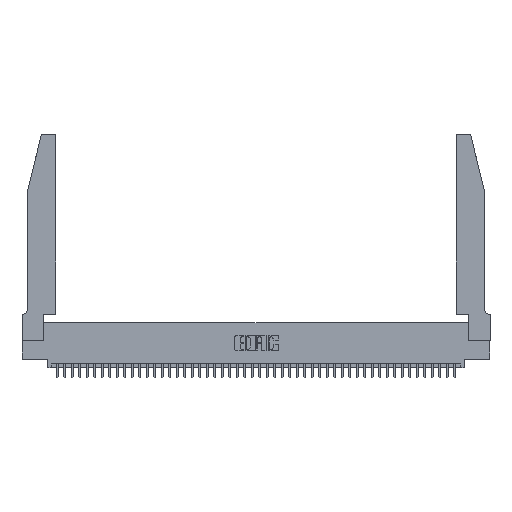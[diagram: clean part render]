
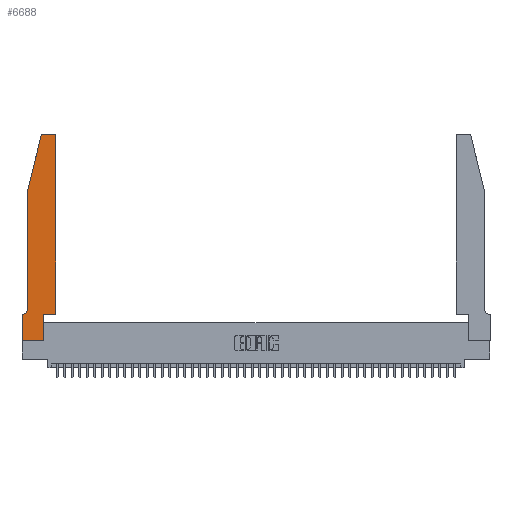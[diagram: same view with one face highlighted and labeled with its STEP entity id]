
A CAD part, top view. The second image highlights one B-rep face of the part: STEP entity #6688.
In plain terms, the highlighted planar face has unit normal (0, 0, 1).
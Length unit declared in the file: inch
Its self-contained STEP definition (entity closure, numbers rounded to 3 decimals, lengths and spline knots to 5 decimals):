
#285 = CARTESIAN_POINT ( 'NONE',  ( 0.0755, 0.35, 0.37 ) ) ;
#939 = VERTEX_POINT ( 'NONE', #20002 ) ;
#1059 = VERTEX_POINT ( 'NONE', #38170 ) ;
#1224 = DIRECTION ( 'NONE',  ( 1., 0., 0. ) ) ;
#1746 = DIRECTION ( 'NONE',  ( 0., -1., 0. ) ) ;
#1923 = VERTEX_POINT ( 'NONE', #30181 ) ;
#2543 = DIRECTION ( 'NONE',  ( 0., 0., 1. ) ) ;
#3639 = CARTESIAN_POINT ( 'NONE',  ( 0.4505, 0.35, 0.37 ) ) ;
#5218 = CARTESIAN_POINT ( 'NONE',  ( 0., 0., 0.37 ) ) ;
#5653 = CARTESIAN_POINT ( 'NONE',  ( 0., 0.35, 0.37 ) ) ;
#5811 = EDGE_CURVE ( 'NONE', #19131, #30120, #33323, .T. ) ;
#5924 = VECTOR ( 'NONE', #8191, 39.37008 ) ;
#6091 = DIRECTION ( 'NONE',  ( 1., 0., 0. ) ) ;
#6151 = EDGE_CURVE ( 'NONE', #26270, #1059, #14539, .T. ) ;
#6517 = CARTESIAN_POINT ( 'NONE',  ( 0.284, 2.75, 0.37 ) ) ;
#6688 = ADVANCED_FACE ( 'NONE', ( #35357 ), #9318, .T. ) ;
#7114 = CARTESIAN_POINT ( 'NONE',  ( 0.0055, 0.42, 0.37 ) ) ;
#7132 = EDGE_CURVE ( 'NONE', #28890, #1923, #33712, .T. ) ;
#7507 = VECTOR ( 'NONE', #43722, 39.37008 ) ;
#7751 = ORIENTED_EDGE ( 'NONE', *, *, #31912, .T. ) ;
#8060 = ORIENTED_EDGE ( 'NONE', *, *, #38276, .T. ) ;
#8191 = DIRECTION ( 'NONE',  ( -1., 0., 0. ) ) ;
#8782 = CARTESIAN_POINT ( 'NONE',  ( 0., 0.35, 0.37 ) ) ;
#8792 = CARTESIAN_POINT ( 'NONE',  ( 0.4505, 2.72, 0.37 ) ) ;
#9318 = PLANE ( 'NONE',  #44135 ) ;
#9440 = VERTEX_POINT ( 'NONE', #23619 ) ;
#10139 = ORIENTED_EDGE ( 'NONE', *, *, #34763, .T. ) ;
#10214 = EDGE_CURVE ( 'NONE', #1923, #26270, #35116, .T. ) ;
#10423 = EDGE_CURVE ( 'NONE', #27678, #28890, #35073, .T. ) ;
#11767 = EDGE_CURVE ( 'NONE', #939, #9440, #40480, .T. ) ;
#12147 = CARTESIAN_POINT ( 'NONE',  ( 0.0755, 2., 0.37 ) ) ;
#13670 = ORIENTED_EDGE ( 'NONE', *, *, #6151, .T. ) ;
#13792 = CARTESIAN_POINT ( 'NONE',  ( 0.0755, 2., 0.37 ) ) ;
#14059 = VERTEX_POINT ( 'NONE', #31666 ) ;
#14539 = CIRCLE ( 'NONE', #23484, 0.03 ) ;
#14559 = VECTOR ( 'NONE', #45145, 39.37008 ) ;
#15178 = ORIENTED_EDGE ( 'NONE', *, *, #5811, .T. ) ;
#15927 = VECTOR ( 'NONE', #21451, 39.37008 ) ;
#16009 = CARTESIAN_POINT ( 'NONE',  ( 0.4505, 0.35, 0.37 ) ) ;
#16106 = ORIENTED_EDGE ( 'NONE', *, *, #28439, .T. ) ;
#16260 = VERTEX_POINT ( 'NONE', #8782 ) ;
#18683 = CARTESIAN_POINT ( 'NONE',  ( 0.2605, 2.75, 0.37 ) ) ;
#19131 = VERTEX_POINT ( 'NONE', #13792 ) ;
#19413 = LINE ( 'NONE', #33968, #29891 ) ;
#20002 = CARTESIAN_POINT ( 'NONE',  ( 0.2865, 0., 0.37 ) ) ;
#21451 = DIRECTION ( 'NONE',  ( -1., 0., 0. ) ) ;
#21618 = CARTESIAN_POINT ( 'NONE',  ( 0.0755, 0.42, 0.37 ) ) ;
#22291 = ORIENTED_EDGE ( 'NONE', *, *, #35395, .T. ) ;
#23072 = LINE ( 'NONE', #285, #15927 ) ;
#23484 = AXIS2_PLACEMENT_3D ( 'NONE', #33943, #44128, #33631 ) ;
#23619 = CARTESIAN_POINT ( 'NONE',  ( 0.2865, 0.35, 0.37 ) ) ;
#23837 = ORIENTED_EDGE ( 'NONE', *, *, #11767, .T. ) ;
#24002 = VECTOR ( 'NONE', #1746, 39.37008 ) ;
#24537 = VECTOR ( 'NONE', #1224, 39.37008 ) ;
#26270 = VERTEX_POINT ( 'NONE', #6517 ) ;
#27308 = LINE ( 'NONE', #44325, #24002 ) ;
#27610 = AXIS2_PLACEMENT_3D ( 'NONE', #34279, #44923, #44320 ) ;
#27678 = VERTEX_POINT ( 'NONE', #16009 ) ;
#28036 = DIRECTION ( 'NONE',  ( 0., 1., 0. ) ) ;
#28439 = EDGE_CURVE ( 'NONE', #9440, #27678, #19413, .T. ) ;
#28890 = VERTEX_POINT ( 'NONE', #8792 ) ;
#29891 = VECTOR ( 'NONE', #6091, 39.37008 ) ;
#30120 = VERTEX_POINT ( 'NONE', #21618 ) ;
#30181 = CARTESIAN_POINT ( 'NONE',  ( 0.4205, 2.75, 0.37 ) ) ;
#30322 = DIRECTION ( 'NONE',  ( 1., 0., 0. ) ) ;
#31113 = VECTOR ( 'NONE', #28036, 39.37008 ) ;
#31170 = DIRECTION ( 'NONE',  ( -1., 0., 0. ) ) ;
#31219 = VERTEX_POINT ( 'NONE', #5218 ) ;
#31666 = CARTESIAN_POINT ( 'NONE',  ( 0.0055, 0.35, 0.37 ) ) ;
#31912 = EDGE_CURVE ( 'NONE', #16260, #31219, #27308, .T. ) ;
#32095 = ORIENTED_EDGE ( 'NONE', *, *, #7132, .T. ) ;
#32753 = EDGE_LOOP ( 'NONE', ( #36867, #13670, #22291, #15178, #41828, #8060, #7751, #10139, #23837, #16106, #40941, #32095 ) ) ;
#33323 = LINE ( 'NONE', #38199, #14559 ) ;
#33509 = CARTESIAN_POINT ( 'NONE',  ( 0., 0., 0.37 ) ) ;
#33631 = DIRECTION ( 'NONE',  ( 1., 0., 0. ) ) ;
#33712 = CIRCLE ( 'NONE', #27610, 0.03 ) ;
#33943 = CARTESIAN_POINT ( 'NONE',  ( 0.284, 2.72, 0.37 ) ) ;
#33968 = CARTESIAN_POINT ( 'NONE',  ( 0.4505, 0.35, 0.37 ) ) ;
#34279 = CARTESIAN_POINT ( 'NONE',  ( 0.4205, 2.72, 0.37 ) ) ;
#34763 = EDGE_CURVE ( 'NONE', #31219, #939, #39389, .T. ) ;
#34986 = CIRCLE ( 'NONE', #44328, 0.07 ) ;
#35073 = LINE ( 'NONE', #3639, #7507 ) ;
#35116 = LINE ( 'NONE', #18683, #5924 ) ;
#35357 = FACE_OUTER_BOUND ( 'NONE', #32753, .T. ) ;
#35395 = EDGE_CURVE ( 'NONE', #1059, #19131, #38814, .T. ) ;
#35697 = CARTESIAN_POINT ( 'NONE',  ( 0.2865, 0.35, 0.37 ) ) ;
#36551 = VECTOR ( 'NONE', #40372, 39.37008 ) ;
#36867 = ORIENTED_EDGE ( 'NONE', *, *, #10214, .T. ) ;
#38170 = CARTESIAN_POINT ( 'NONE',  ( 0.25487, 2.72718, 0.37 ) ) ;
#38199 = CARTESIAN_POINT ( 'NONE',  ( 0.0755, 2., 0.37 ) ) ;
#38276 = EDGE_CURVE ( 'NONE', #14059, #16260, #23072, .T. ) ;
#38814 = LINE ( 'NONE', #12147, #36551 ) ;
#38861 = DIRECTION ( 'NONE',  ( 0., 0., -1. ) ) ;
#39389 = LINE ( 'NONE', #33509, #24537 ) ;
#40201 = EDGE_CURVE ( 'NONE', #30120, #14059, #34986, .T. ) ;
#40372 = DIRECTION ( 'NONE',  ( -0.239, -0.971, 0. ) ) ;
#40480 = LINE ( 'NONE', #35697, #31113 ) ;
#40941 = ORIENTED_EDGE ( 'NONE', *, *, #10423, .T. ) ;
#41828 = ORIENTED_EDGE ( 'NONE', *, *, #40201, .T. ) ;
#43722 = DIRECTION ( 'NONE',  ( 0., 1., 0. ) ) ;
#44128 = DIRECTION ( 'NONE',  ( 0., 0., 1. ) ) ;
#44135 = AXIS2_PLACEMENT_3D ( 'NONE', #5653, #2543, #30322 ) ;
#44320 = DIRECTION ( 'NONE',  ( 1., 0., 0. ) ) ;
#44325 = CARTESIAN_POINT ( 'NONE',  ( 0., 0., 0.37 ) ) ;
#44328 = AXIS2_PLACEMENT_3D ( 'NONE', #7114, #38861, #31170 ) ;
#44923 = DIRECTION ( 'NONE',  ( 0., 0., 1. ) ) ;
#45145 = DIRECTION ( 'NONE',  ( 0., -1., 0. ) ) ;
